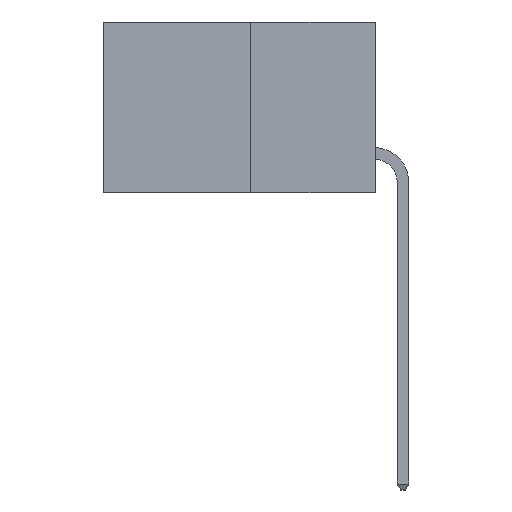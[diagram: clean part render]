
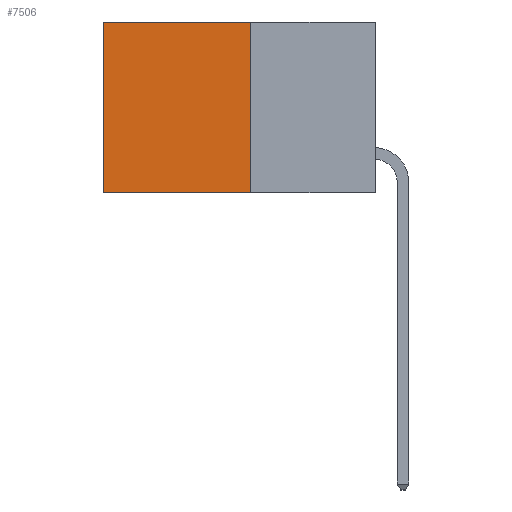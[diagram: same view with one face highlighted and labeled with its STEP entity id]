
A CAD part, left-side view. The second image highlights one B-rep face of the part: STEP entity #7506.
In plain terms, the highlighted planar face has unit normal (-1, 0, 0).
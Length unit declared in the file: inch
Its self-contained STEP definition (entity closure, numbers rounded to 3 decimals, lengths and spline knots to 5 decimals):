
#344 = VERTEX_POINT ( 'NONE', #8928 ) ;
#401 = VECTOR ( 'NONE', #2477, 39.37008 ) ;
#770 = AXIS2_PLACEMENT_3D ( 'NONE', #5123, #12869, #6278 ) ;
#1214 = ORIENTED_EDGE ( 'NONE', *, *, #7687, .T. ) ;
#1264 = FACE_OUTER_BOUND ( 'NONE', #1609, .T. ) ;
#1449 = LINE ( 'NONE', #14255, #4697 ) ;
#1609 = EDGE_LOOP ( 'NONE', ( #5366, #11071, #7473, #1214 ) ) ;
#2477 = DIRECTION ( 'NONE',  ( 0., 0., -1. ) ) ;
#2532 = CARTESIAN_POINT ( 'NONE',  ( 0.277, 0.27, -0.37 ) ) ;
#3083 = CARTESIAN_POINT ( 'NONE',  ( 0.277, 0.59, 0. ) ) ;
#3366 = DIRECTION ( 'NONE',  ( 0., 0., -1. ) ) ;
#3906 = CARTESIAN_POINT ( 'NONE',  ( 0.277, 0.27, -0.37 ) ) ;
#4068 = LINE ( 'NONE', #8349, #401 ) ;
#4287 = DIRECTION ( 'NONE',  ( 0., 1., 0. ) ) ;
#4697 = VECTOR ( 'NONE', #4287, 39.37008 ) ;
#5123 = CARTESIAN_POINT ( 'NONE',  ( 0.277, 0.27, -0.37 ) ) ;
#5366 = ORIENTED_EDGE ( 'NONE', *, *, #14150, .T. ) ;
#5613 = VECTOR ( 'NONE', #12742, 39.37008 ) ;
#5738 = CARTESIAN_POINT ( 'NONE',  ( 0.277, 0.59, -0.37 ) ) ;
#6278 = DIRECTION ( 'NONE',  ( 0., 0., -1. ) ) ;
#7021 = VERTEX_POINT ( 'NONE', #3906 ) ;
#7464 = VECTOR ( 'NONE', #3366, 39.37008 ) ;
#7473 = ORIENTED_EDGE ( 'NONE', *, *, #11302, .F. ) ;
#7506 = ADVANCED_FACE ( 'NONE', ( #1264 ), #11812, .F. ) ;
#7687 = EDGE_CURVE ( 'NONE', #8426, #14645, #1449, .T. ) ;
#8293 = LINE ( 'NONE', #2532, #5613 ) ;
#8349 = CARTESIAN_POINT ( 'NONE',  ( 0.277, 0.27, -0.37 ) ) ;
#8426 = VERTEX_POINT ( 'NONE', #10091 ) ;
#8689 = EDGE_CURVE ( 'NONE', #7021, #344, #8293, .T. ) ;
#8928 = CARTESIAN_POINT ( 'NONE',  ( 0.277, 0.59, -0.37 ) ) ;
#9699 = LINE ( 'NONE', #5738, #7464 ) ;
#10091 = CARTESIAN_POINT ( 'NONE',  ( 0.277, 0.27, 0. ) ) ;
#11071 = ORIENTED_EDGE ( 'NONE', *, *, #8689, .F. ) ;
#11302 = EDGE_CURVE ( 'NONE', #8426, #7021, #4068, .T. ) ;
#11812 = PLANE ( 'NONE',  #770 ) ;
#12742 = DIRECTION ( 'NONE',  ( 0., 1., 0. ) ) ;
#12869 = DIRECTION ( 'NONE',  ( 1., 0., 0. ) ) ;
#14150 = EDGE_CURVE ( 'NONE', #14645, #344, #9699, .T. ) ;
#14255 = CARTESIAN_POINT ( 'NONE',  ( 0.277, 0.27, 0. ) ) ;
#14645 = VERTEX_POINT ( 'NONE', #3083 ) ;
